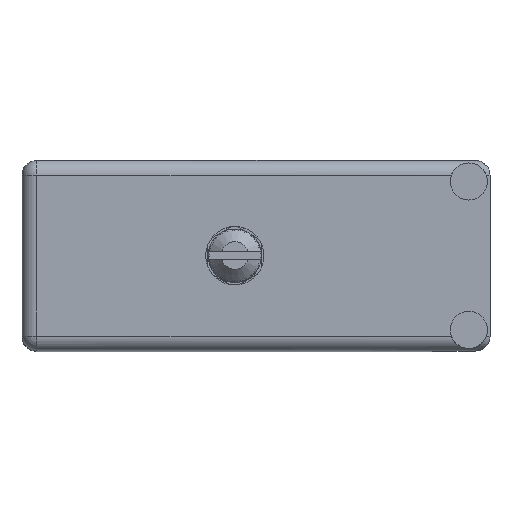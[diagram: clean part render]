
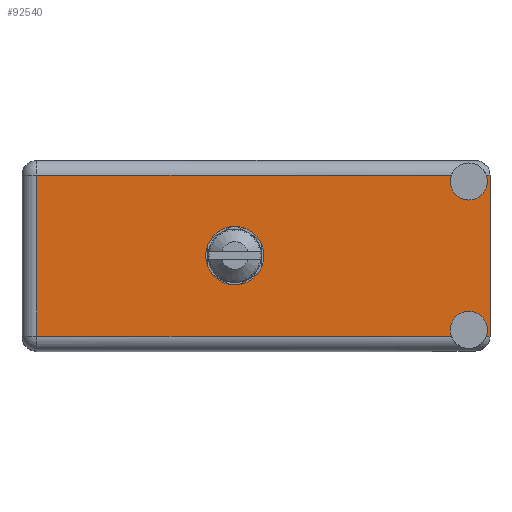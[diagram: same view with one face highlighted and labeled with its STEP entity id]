
A CAD part, top view. The second image highlights one B-rep face of the part: STEP entity #92540.
In plain terms, the highlighted face is planar.
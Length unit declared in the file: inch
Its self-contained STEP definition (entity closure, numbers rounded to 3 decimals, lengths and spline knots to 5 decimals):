
#253 = CARTESIAN_POINT ( 'NONE',  ( 2.02562, 1.566, -0.829 ) ) ;
#3597 = PLANE ( 'NONE',  #24461 ) ;
#4366 = EDGE_CURVE ( 'NONE', #4724, #16382, #8197, .T. ) ;
#4411 = ORIENTED_EDGE ( 'NONE', *, *, #13916, .F. ) ;
#4724 = VERTEX_POINT ( 'NONE', #106201 ) ;
#5758 = CARTESIAN_POINT ( 'NONE',  ( 2.19038, 1.566, -0.829 ) ) ;
#6820 = VECTOR ( 'NONE', #95908, 39.37008 ) ;
#7579 = CARTESIAN_POINT ( 'NONE',  ( 0.07, 1.566, -0.07 ) ) ;
#7689 = EDGE_CURVE ( 'NONE', #56583, #111987, #13570, .T. ) ;
#7973 = CARTESIAN_POINT ( 'NONE',  ( 2.108, 1.566, -0.187 ) ) ;
#8197 = CIRCLE ( 'NONE', #75597, 0.0875 ) ;
#8751 = ORIENTED_EDGE ( 'NONE', *, *, #7689, .T. ) ;
#9143 = CIRCLE ( 'NONE', #12826, 0.1375 ) ;
#9739 = ORIENTED_EDGE ( 'NONE', *, *, #11250, .T. ) ;
#11250 = EDGE_CURVE ( 'NONE', #4724, #84922, #87910, .T. ) ;
#11600 = FACE_BOUND ( 'NONE', #87319, .T. ) ;
#12169 = DIRECTION ( 'NONE',  ( 0., 1., 0. ) ) ;
#12826 = AXIS2_PLACEMENT_3D ( 'NONE', #32549, #31986, #49627 ) ;
#13562 = ORIENTED_EDGE ( 'NONE', *, *, #64925, .T. ) ;
#13570 = LINE ( 'NONE', #64937, #74287 ) ;
#13916 = EDGE_CURVE ( 'NONE', #66403, #57178, #103745, .T. ) ;
#14771 = CARTESIAN_POINT ( 'NONE',  ( 2.108, 1.566, -0.0995 ) ) ;
#15696 = LINE ( 'NONE', #48817, #46042 ) ;
#15994 = CARTESIAN_POINT ( 'NONE',  ( 2.208, 1.566, -0.07 ) ) ;
#16118 = EDGE_CURVE ( 'NONE', #35112, #66403, #83940, .T. ) ;
#16382 = VERTEX_POINT ( 'NONE', #7973 ) ;
#20852 = DIRECTION ( 'NONE',  ( 0., 0., 1. ) ) ;
#21282 = CARTESIAN_POINT ( 'NONE',  ( 2.02562, 1.566, -0.07 ) ) ;
#21299 = CARTESIAN_POINT ( 'NONE',  ( 1.004, 1.566, -0.587 ) ) ;
#23688 = DIRECTION ( 'NONE',  ( -1., 0., 0. ) ) ;
#24461 = AXIS2_PLACEMENT_3D ( 'NONE', #28163, #12169, #108085 ) ;
#24632 = ORIENTED_EDGE ( 'NONE', *, *, #112109, .F. ) ;
#25913 = ORIENTED_EDGE ( 'NONE', *, *, #26205, .T. ) ;
#26205 = EDGE_CURVE ( 'NONE', #63522, #57178, #15696, .T. ) ;
#27983 = ORIENTED_EDGE ( 'NONE', *, *, #73467, .F. ) ;
#28163 = CARTESIAN_POINT ( 'NONE',  ( 0., 1.566, -0.899 ) ) ;
#28509 = DIRECTION ( 'NONE',  ( 0., 0., 1. ) ) ;
#30872 = DIRECTION ( 'NONE',  ( 1., 0., 0. ) ) ;
#31986 = DIRECTION ( 'NONE',  ( 0., 1., 0. ) ) ;
#32549 = CARTESIAN_POINT ( 'NONE',  ( 1.004, 1.566, -0.4495 ) ) ;
#32899 = VERTEX_POINT ( 'NONE', #106007 ) ;
#33420 = CARTESIAN_POINT ( 'NONE',  ( 0.07, 1.566, -0.829 ) ) ;
#35112 = VERTEX_POINT ( 'NONE', #253 ) ;
#35170 = LINE ( 'NONE', #43733, #112330 ) ;
#35696 = DIRECTION ( 'NONE',  ( 0., 1., 0. ) ) ;
#36729 = FACE_OUTER_BOUND ( 'NONE', #44883, .T. ) ;
#38005 = CARTESIAN_POINT ( 'NONE',  ( 2.108, 1.566, -0.7995 ) ) ;
#39049 = VECTOR ( 'NONE', #30872, 39.37008 ) ;
#41919 = AXIS2_PLACEMENT_3D ( 'NONE', #14771, #59276, #76434 ) ;
#43733 = CARTESIAN_POINT ( 'NONE',  ( 0., 1.566, -0.829 ) ) ;
#44883 = EDGE_LOOP ( 'NONE', ( #61463, #108955, #46920, #9739, #24632, #25913, #4411, #105363, #13562, #8751 ) ) ;
#45689 = ORIENTED_EDGE ( 'NONE', *, *, #109536, .F. ) ;
#46042 = VECTOR ( 'NONE', #23688, 39.37008 ) ;
#46920 = ORIENTED_EDGE ( 'NONE', *, *, #4366, .F. ) ;
#47587 = VECTOR ( 'NONE', #99418, 39.37008 ) ;
#48817 = CARTESIAN_POINT ( 'NONE',  ( 0., 1.566, -0.829 ) ) ;
#49456 = CARTESIAN_POINT ( 'NONE',  ( 2.108, 1.566, -0.7995 ) ) ;
#49627 = DIRECTION ( 'NONE',  ( 0., 0., 1. ) ) ;
#53359 = DIRECTION ( 'NONE',  ( 0., 0., 1. ) ) ;
#54441 = AXIS2_PLACEMENT_3D ( 'NONE', #38005, #64242, #20852 ) ;
#56583 = VERTEX_POINT ( 'NONE', #33420 ) ;
#57178 = VERTEX_POINT ( 'NONE', #5758 ) ;
#57650 = LINE ( 'NONE', #109646, #39049 ) ;
#58040 = CIRCLE ( 'NONE', #61734, 0.1375 ) ;
#58981 = CARTESIAN_POINT ( 'NONE',  ( 2.208, 1.566, -0.829 ) ) ;
#59276 = DIRECTION ( 'NONE',  ( 0., 1., 0. ) ) ;
#61190 = VERTEX_POINT ( 'NONE', #21282 ) ;
#61463 = ORIENTED_EDGE ( 'NONE', *, *, #92963, .T. ) ;
#61734 = AXIS2_PLACEMENT_3D ( 'NONE', #106737, #107880, #28509 ) ;
#63522 = VERTEX_POINT ( 'NONE', #58981 ) ;
#64242 = DIRECTION ( 'NONE',  ( 0., 1., 0. ) ) ;
#64925 = EDGE_CURVE ( 'NONE', #35112, #56583, #35170, .T. ) ;
#64937 = CARTESIAN_POINT ( 'NONE',  ( 0.07, 1.566, -0.899 ) ) ;
#66403 = VERTEX_POINT ( 'NONE', #104004 ) ;
#73141 = LINE ( 'NONE', #90312, #47587 ) ;
#73467 = EDGE_CURVE ( 'NONE', #32899, #95179, #58040, .T. ) ;
#74287 = VECTOR ( 'NONE', #110046, 39.37008 ) ;
#75597 = AXIS2_PLACEMENT_3D ( 'NONE', #112824, #35696, #53359 ) ;
#76434 = DIRECTION ( 'NONE',  ( 0., 0., 1. ) ) ;
#77086 = EDGE_CURVE ( 'NONE', #16382, #61190, #111213, .T. ) ;
#82084 = DIRECTION ( 'NONE',  ( 0., 1., 0. ) ) ;
#83940 = CIRCLE ( 'NONE', #107632, 0.0875 ) ;
#84922 = VERTEX_POINT ( 'NONE', #108724 ) ;
#87319 = EDGE_LOOP ( 'NONE', ( #27983, #45689 ) ) ;
#87910 = LINE ( 'NONE', #15994, #6820 ) ;
#90312 = CARTESIAN_POINT ( 'NONE',  ( 2.208, 1.566, 0. ) ) ;
#92540 = ADVANCED_FACE ( 'NONE', ( #11600, #36729 ), #3597, .T. ) ;
#92963 = EDGE_CURVE ( 'NONE', #111987, #61190, #57650, .T. ) ;
#95179 = VERTEX_POINT ( 'NONE', #21299 ) ;
#95908 = DIRECTION ( 'NONE',  ( 1., 0., 0. ) ) ;
#99418 = DIRECTION ( 'NONE',  ( 0., 0., 1. ) ) ;
#103745 = CIRCLE ( 'NONE', #54441, 0.0875 ) ;
#104004 = CARTESIAN_POINT ( 'NONE',  ( 2.108, 1.566, -0.712 ) ) ;
#104835 = DIRECTION ( 'NONE',  ( -1., 0., 0. ) ) ;
#105363 = ORIENTED_EDGE ( 'NONE', *, *, #16118, .F. ) ;
#106007 = CARTESIAN_POINT ( 'NONE',  ( 1.004, 1.566, -0.312 ) ) ;
#106201 = CARTESIAN_POINT ( 'NONE',  ( 2.19038, 1.566, -0.07 ) ) ;
#106737 = CARTESIAN_POINT ( 'NONE',  ( 1.004, 1.566, -0.4495 ) ) ;
#107632 = AXIS2_PLACEMENT_3D ( 'NONE', #49456, #82084, #111048 ) ;
#107880 = DIRECTION ( 'NONE',  ( 0., 1., 0. ) ) ;
#108085 = DIRECTION ( 'NONE',  ( 0., 0., 1. ) ) ;
#108724 = CARTESIAN_POINT ( 'NONE',  ( 2.208, 1.566, -0.07 ) ) ;
#108955 = ORIENTED_EDGE ( 'NONE', *, *, #77086, .F. ) ;
#109536 = EDGE_CURVE ( 'NONE', #95179, #32899, #9143, .T. ) ;
#109646 = CARTESIAN_POINT ( 'NONE',  ( 2.208, 1.566, -0.07 ) ) ;
#110046 = DIRECTION ( 'NONE',  ( 0., 0., 1. ) ) ;
#111048 = DIRECTION ( 'NONE',  ( 0., 0., 1. ) ) ;
#111213 = CIRCLE ( 'NONE', #41919, 0.0875 ) ;
#111987 = VERTEX_POINT ( 'NONE', #7579 ) ;
#112109 = EDGE_CURVE ( 'NONE', #63522, #84922, #73141, .T. ) ;
#112330 = VECTOR ( 'NONE', #104835, 39.37008 ) ;
#112824 = CARTESIAN_POINT ( 'NONE',  ( 2.108, 1.566, -0.0995 ) ) ;
